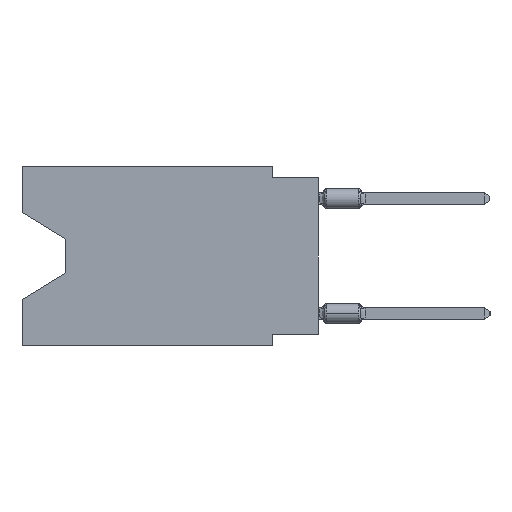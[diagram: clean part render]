
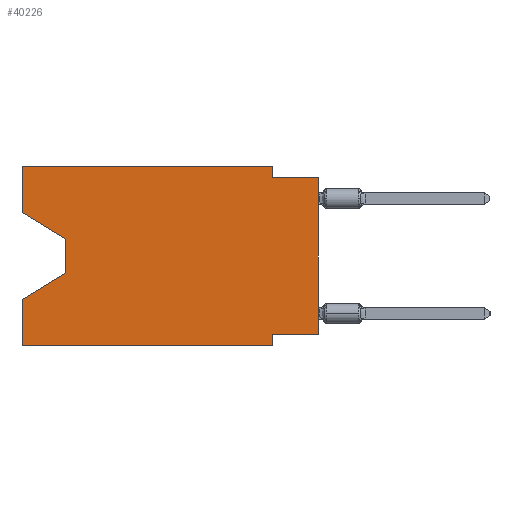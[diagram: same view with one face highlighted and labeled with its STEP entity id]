
A CAD part, left-side view. The second image highlights one B-rep face of the part: STEP entity #40226.
In plain terms, the highlighted planar face has unit normal (-1, 0, 0).
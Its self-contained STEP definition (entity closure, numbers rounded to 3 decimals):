
#46 = CARTESIAN_POINT ( 'NONE',  ( 0., 2.54, -9.906 ) ) ;
#87 = VERTEX_POINT ( 'NONE', #53814 ) ;
#649 = EDGE_CURVE ( 'NONE', #29425, #12689, #6234, .T. ) ;
#796 = EDGE_CURVE ( 'NONE', #33574, #12689, #22247, .T. ) ;
#4486 = CARTESIAN_POINT ( 'NONE',  ( 0., 2.54, -9.271 ) ) ;
#4701 = LINE ( 'NONE', #19475, #17592 ) ;
#5646 = CARTESIAN_POINT ( 'NONE',  ( 0., 0., -9.271 ) ) ;
#6234 = LINE ( 'NONE', #11054, #56360 ) ;
#8298 = CARTESIAN_POINT ( 'NONE',  ( 0., 16.383, 0. ) ) ;
#8478 = LINE ( 'NONE', #57600, #38729 ) ;
#8562 = CARTESIAN_POINT ( 'NONE',  ( 0., 0., -9.271 ) ) ;
#8585 = ORIENTED_EDGE ( 'NONE', *, *, #23607, .T. ) ;
#8745 = ORIENTED_EDGE ( 'NONE', *, *, #11303, .T. ) ;
#9829 = DIRECTION ( 'NONE',  ( 0., -1., 0. ) ) ;
#10379 = LINE ( 'NONE', #59819, #17187 ) ;
#10612 = CARTESIAN_POINT ( 'NONE',  ( 0., 16.383, 0. ) ) ;
#10702 = VECTOR ( 'NONE', #55002, 1000. ) ;
#11054 = CARTESIAN_POINT ( 'NONE',  ( 0., 13.97, -5.893 ) ) ;
#11061 = CARTESIAN_POINT ( 'NONE',  ( 0., 16.383, 0. ) ) ;
#11303 = EDGE_CURVE ( 'NONE', #21145, #35255, #10379, .T. ) ;
#12103 = EDGE_CURVE ( 'NONE', #41922, #23719, #49941, .T. ) ;
#12689 = VERTEX_POINT ( 'NONE', #54377 ) ;
#14298 = EDGE_LOOP ( 'NONE', ( #8745, #17738, #18490, #49383, #36614, #30616, #63292, #8585, #22344, #52011, #46996, #15359 ) ) ;
#14338 = DIRECTION ( 'NONE',  ( 0., 0., -1. ) ) ;
#14624 = VERTEX_POINT ( 'NONE', #4486 ) ;
#15359 = ORIENTED_EDGE ( 'NONE', *, *, #33389, .F. ) ;
#15436 = FACE_OUTER_BOUND ( 'NONE', #14298, .T. ) ;
#15452 = DIRECTION ( 'NONE',  ( 0., -1., 0. ) ) ;
#16229 = VECTOR ( 'NONE', #14338, 1000. ) ;
#17187 = VECTOR ( 'NONE', #20992, 1000. ) ;
#17592 = VECTOR ( 'NONE', #48034, 1000. ) ;
#17738 = ORIENTED_EDGE ( 'NONE', *, *, #30170, .T. ) ;
#18490 = ORIENTED_EDGE ( 'NONE', *, *, #649, .T. ) ;
#19475 = CARTESIAN_POINT ( 'NONE',  ( 0., 13.97, -4.013 ) ) ;
#19924 = DIRECTION ( 'NONE',  ( 1., 0., 0. ) ) ;
#20374 = LINE ( 'NONE', #11061, #63167 ) ;
#20759 = DIRECTION ( 'NONE',  ( 0., 0., -1. ) ) ;
#20992 = DIRECTION ( 'NONE',  ( 0., -0.855, -0.519 ) ) ;
#21145 = VERTEX_POINT ( 'NONE', #52633 ) ;
#22247 = LINE ( 'NONE', #41834, #62527 ) ;
#22344 = ORIENTED_EDGE ( 'NONE', *, *, #51664, .F. ) ;
#23012 = CARTESIAN_POINT ( 'NONE',  ( 0., 2.54, -9.906 ) ) ;
#23306 = EDGE_CURVE ( 'NONE', #14624, #62880, #23629, .T. ) ;
#23607 = EDGE_CURVE ( 'NONE', #42404, #28660, #8478, .T. ) ;
#23629 = LINE ( 'NONE', #23012, #16229 ) ;
#23719 = VERTEX_POINT ( 'NONE', #33503 ) ;
#24100 = LINE ( 'NONE', #28915, #59877 ) ;
#25880 = CARTESIAN_POINT ( 'NONE',  ( 0., 2.54, 0. ) ) ;
#26475 = VECTOR ( 'NONE', #20759, 1000. ) ;
#27569 = LINE ( 'NONE', #8298, #10702 ) ;
#28660 = VERTEX_POINT ( 'NONE', #60283 ) ;
#28915 = CARTESIAN_POINT ( 'NONE',  ( 0., 16.383, -9.906 ) ) ;
#29425 = VERTEX_POINT ( 'NONE', #62412 ) ;
#29659 = DIRECTION ( 'NONE',  ( 0., -1., 0. ) ) ;
#30170 = EDGE_CURVE ( 'NONE', #35255, #29425, #4701, .T. ) ;
#30616 = ORIENTED_EDGE ( 'NONE', *, *, #23306, .F. ) ;
#32305 = LINE ( 'NONE', #8562, #59070 ) ;
#33389 = EDGE_CURVE ( 'NONE', #21145, #87, #27569, .T. ) ;
#33503 = CARTESIAN_POINT ( 'NONE',  ( 0., 2.54, -0.635 ) ) ;
#33574 = VERTEX_POINT ( 'NONE', #33661 ) ;
#33661 = CARTESIAN_POINT ( 'NONE',  ( 0., 16.383, -9.906 ) ) ;
#35255 = VERTEX_POINT ( 'NONE', #52764 ) ;
#36614 = ORIENTED_EDGE ( 'NONE', *, *, #57063, .T. ) ;
#37511 = EDGE_CURVE ( 'NONE', #42404, #14624, #32305, .T. ) ;
#38729 = VECTOR ( 'NONE', #43479, 1000. ) ;
#38784 = CARTESIAN_POINT ( 'NONE',  ( 0., 2.54, 0. ) ) ;
#40226 = ADVANCED_FACE ( 'NONE', ( #15436 ), #53618, .F. ) ;
#41834 = CARTESIAN_POINT ( 'NONE',  ( 0., 16.383, 0. ) ) ;
#41922 = VERTEX_POINT ( 'NONE', #38784 ) ;
#42404 = VERTEX_POINT ( 'NONE', #5646 ) ;
#42595 = DIRECTION ( 'NONE',  ( 0., 1., 0. ) ) ;
#43479 = DIRECTION ( 'NONE',  ( 0., 0., 1. ) ) ;
#46494 = VECTOR ( 'NONE', #9829, 1000. ) ;
#46991 = AXIS2_PLACEMENT_3D ( 'NONE', #10612, #19924, #53305 ) ;
#46996 = ORIENTED_EDGE ( 'NONE', *, *, #62134, .F. ) ;
#48034 = DIRECTION ( 'NONE',  ( 0., 0., -1. ) ) ;
#49383 = ORIENTED_EDGE ( 'NONE', *, *, #796, .F. ) ;
#49941 = LINE ( 'NONE', #25880, #26475 ) ;
#51664 = EDGE_CURVE ( 'NONE', #23719, #28660, #54775, .T. ) ;
#52011 = ORIENTED_EDGE ( 'NONE', *, *, #12103, .F. ) ;
#52633 = CARTESIAN_POINT ( 'NONE',  ( 0., 16.383, -2.546 ) ) ;
#52764 = CARTESIAN_POINT ( 'NONE',  ( 0., 13.97, -4.013 ) ) ;
#53305 = DIRECTION ( 'NONE',  ( 0., 0., -1. ) ) ;
#53482 = CARTESIAN_POINT ( 'NONE',  ( 0., 0., -0.635 ) ) ;
#53618 = PLANE ( 'NONE',  #46991 ) ;
#53814 = CARTESIAN_POINT ( 'NONE',  ( 0., 16.383, 0. ) ) ;
#54377 = CARTESIAN_POINT ( 'NONE',  ( 0., 16.383, -7.36 ) ) ;
#54775 = LINE ( 'NONE', #53482, #46494 ) ;
#55002 = DIRECTION ( 'NONE',  ( 0., 0., 1. ) ) ;
#56360 = VECTOR ( 'NONE', #60781, 1000. ) ;
#57063 = EDGE_CURVE ( 'NONE', #33574, #62880, #24100, .T. ) ;
#57600 = CARTESIAN_POINT ( 'NONE',  ( 0., 0., 0. ) ) ;
#59070 = VECTOR ( 'NONE', #42595, 1000. ) ;
#59819 = CARTESIAN_POINT ( 'NONE',  ( 0., 16.383, -2.546 ) ) ;
#59877 = VECTOR ( 'NONE', #15452, 1000. ) ;
#60283 = CARTESIAN_POINT ( 'NONE',  ( 0., 0., -0.635 ) ) ;
#60781 = DIRECTION ( 'NONE',  ( 0., 0.855, -0.519 ) ) ;
#62134 = EDGE_CURVE ( 'NONE', #87, #41922, #20374, .T. ) ;
#62354 = DIRECTION ( 'NONE',  ( 0., 0., 1. ) ) ;
#62412 = CARTESIAN_POINT ( 'NONE',  ( 0., 13.97, -5.893 ) ) ;
#62527 = VECTOR ( 'NONE', #62354, 1000. ) ;
#62880 = VERTEX_POINT ( 'NONE', #46 ) ;
#63167 = VECTOR ( 'NONE', #29659, 1000. ) ;
#63292 = ORIENTED_EDGE ( 'NONE', *, *, #37511, .F. ) ;
